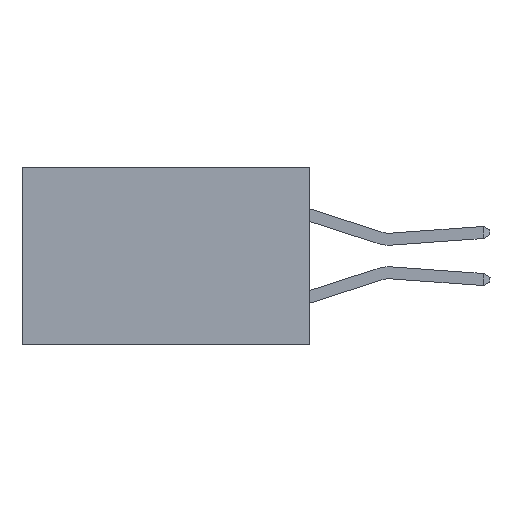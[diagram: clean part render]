
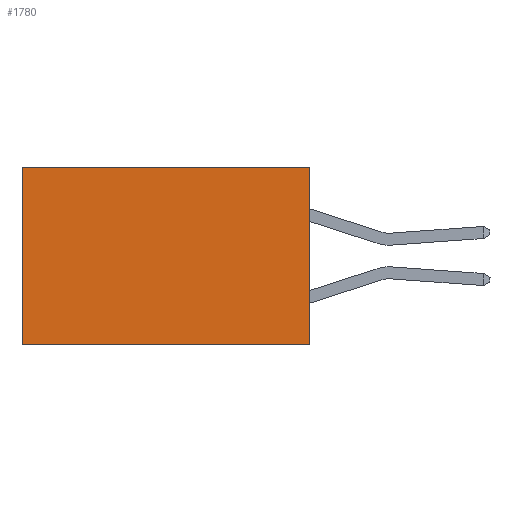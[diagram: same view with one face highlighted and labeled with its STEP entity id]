
A CAD part, left-side view. The second image highlights one B-rep face of the part: STEP entity #1780.
In plain terms, the highlighted planar face has unit normal (-1, 0, 0).
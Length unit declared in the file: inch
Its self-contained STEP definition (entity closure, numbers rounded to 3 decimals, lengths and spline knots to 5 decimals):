
#7 = DIRECTION ( 'NONE',  ( 0., 1., 0. ) ) ;
#628 = LINE ( 'NONE', #12171, #7075 ) ;
#755 = ORIENTED_EDGE ( 'NONE', *, *, #9850, .T. ) ;
#1137 = VECTOR ( 'NONE', #7, 39.37008 ) ;
#1202 = CARTESIAN_POINT ( 'NONE',  ( 0.298, 0.6, -0.37 ) ) ;
#1489 = LINE ( 'NONE', #3106, #7008 ) ;
#1780 = ADVANCED_FACE ( 'NONE', ( #3494 ), #4643, .F. ) ;
#2474 = VERTEX_POINT ( 'NONE', #1202 ) ;
#3106 = CARTESIAN_POINT ( 'NONE',  ( 0.298, 0.6, 0. ) ) ;
#3199 = ORIENTED_EDGE ( 'NONE', *, *, #5836, .T. ) ;
#3343 = ORIENTED_EDGE ( 'NONE', *, *, #3515, .F. ) ;
#3494 = FACE_OUTER_BOUND ( 'NONE', #3883, .T. ) ;
#3515 = EDGE_CURVE ( 'NONE', #9060, #8349, #10899, .T. ) ;
#3776 = CARTESIAN_POINT ( 'NONE',  ( 0.298, 0., 0. ) ) ;
#3883 = EDGE_LOOP ( 'NONE', ( #3199, #9685, #3343, #755 ) ) ;
#4643 = PLANE ( 'NONE',  #6397 ) ;
#5374 = EDGE_CURVE ( 'NONE', #8349, #2474, #6538, .T. ) ;
#5653 = CARTESIAN_POINT ( 'NONE',  ( 0.298, 0., 0. ) ) ;
#5776 = CARTESIAN_POINT ( 'NONE',  ( 0.298, 0., -0.37 ) ) ;
#5836 = EDGE_CURVE ( 'NONE', #9702, #2474, #1489, .T. ) ;
#6397 = AXIS2_PLACEMENT_3D ( 'NONE', #3776, #7700, #12345 ) ;
#6538 = LINE ( 'NONE', #5776, #1137 ) ;
#6599 = CARTESIAN_POINT ( 'NONE',  ( 0.298, 0., 0. ) ) ;
#7008 = VECTOR ( 'NONE', #10561, 39.37008 ) ;
#7075 = VECTOR ( 'NONE', #10288, 39.37008 ) ;
#7369 = CARTESIAN_POINT ( 'NONE',  ( 0.298, 0., -0.37 ) ) ;
#7700 = DIRECTION ( 'NONE',  ( 1., 0., 0. ) ) ;
#8349 = VERTEX_POINT ( 'NONE', #7369 ) ;
#8355 = VECTOR ( 'NONE', #8563, 39.37008 ) ;
#8563 = DIRECTION ( 'NONE',  ( 0., 0., -1. ) ) ;
#9060 = VERTEX_POINT ( 'NONE', #5653 ) ;
#9199 = CARTESIAN_POINT ( 'NONE',  ( 0.298, 0.6, 0. ) ) ;
#9685 = ORIENTED_EDGE ( 'NONE', *, *, #5374, .F. ) ;
#9702 = VERTEX_POINT ( 'NONE', #9199 ) ;
#9850 = EDGE_CURVE ( 'NONE', #9060, #9702, #628, .T. ) ;
#10288 = DIRECTION ( 'NONE',  ( 0., 1., 0. ) ) ;
#10561 = DIRECTION ( 'NONE',  ( 0., 0., -1. ) ) ;
#10899 = LINE ( 'NONE', #6599, #8355 ) ;
#12171 = CARTESIAN_POINT ( 'NONE',  ( 0.298, 0., 0. ) ) ;
#12345 = DIRECTION ( 'NONE',  ( 0., 0., -1. ) ) ;
